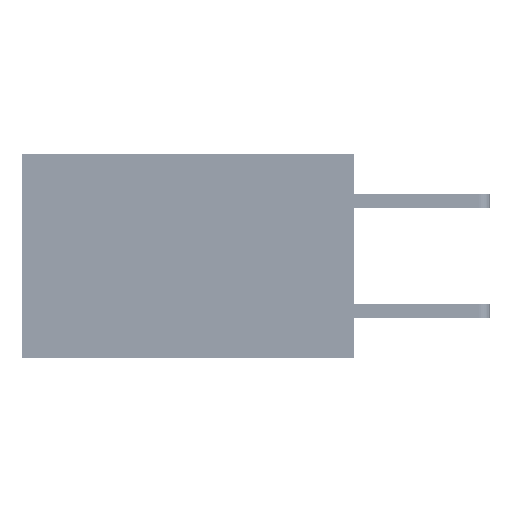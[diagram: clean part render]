
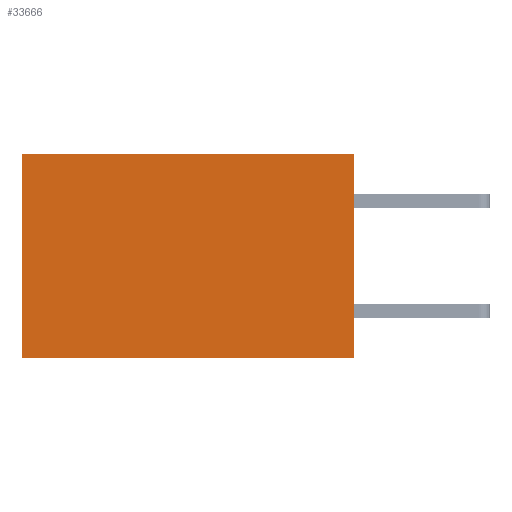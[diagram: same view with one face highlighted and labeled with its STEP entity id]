
A CAD part, left-side view. The second image highlights one B-rep face of the part: STEP entity #33666.
In plain terms, the highlighted planar face has unit normal (-1, 0, 0).
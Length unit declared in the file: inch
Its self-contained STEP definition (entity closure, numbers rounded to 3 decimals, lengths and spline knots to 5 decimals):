
#2239 = EDGE_CURVE ( 'NONE', #25159, #16128, #25951, .T. ) ;
#2943 = AXIS2_PLACEMENT_3D ( 'NONE', #47793, #18213, #14325 ) ;
#3697 = CARTESIAN_POINT ( 'NONE',  ( 0.2875, 0., 0. ) ) ;
#3745 = CARTESIAN_POINT ( 'NONE',  ( 0.2875, 0.6, 0. ) ) ;
#5160 = ORIENTED_EDGE ( 'NONE', *, *, #27192, .T. ) ;
#6220 = VERTEX_POINT ( 'NONE', #3697 ) ;
#8939 = ORIENTED_EDGE ( 'NONE', *, *, #11857, .T. ) ;
#9213 = FACE_OUTER_BOUND ( 'NONE', #27190, .T. ) ;
#11317 = DIRECTION ( 'NONE',  ( 0., 1., 0. ) ) ;
#11857 = EDGE_CURVE ( 'NONE', #6220, #40453, #12612, .T. ) ;
#12612 = LINE ( 'NONE', #37212, #35922 ) ;
#13929 = DIRECTION ( 'NONE',  ( 0., 1., 0. ) ) ;
#14325 = DIRECTION ( 'NONE',  ( 0., 0., -1. ) ) ;
#14468 = VECTOR ( 'NONE', #45276, 39.37008 ) ;
#15050 = CARTESIAN_POINT ( 'NONE',  ( 0.2875, 0., 0. ) ) ;
#16128 = VERTEX_POINT ( 'NONE', #22637 ) ;
#17211 = VECTOR ( 'NONE', #13929, 39.37008 ) ;
#18213 = DIRECTION ( 'NONE',  ( 1., 0., 0. ) ) ;
#21013 = ORIENTED_EDGE ( 'NONE', *, *, #2239, .F. ) ;
#21557 = EDGE_CURVE ( 'NONE', #6220, #25159, #22642, .T. ) ;
#22637 = CARTESIAN_POINT ( 'NONE',  ( 0.2875, 0.6, -0.37 ) ) ;
#22642 = LINE ( 'NONE', #15050, #14468 ) ;
#25159 = VERTEX_POINT ( 'NONE', #44171 ) ;
#25951 = LINE ( 'NONE', #40443, #17211 ) ;
#27190 = EDGE_LOOP ( 'NONE', ( #5160, #21013, #37484, #8939 ) ) ;
#27192 = EDGE_CURVE ( 'NONE', #40453, #16128, #34489, .T. ) ;
#29317 = PLANE ( 'NONE',  #2943 ) ;
#33666 = ADVANCED_FACE ( 'NONE', ( #9213 ), #29317, .F. ) ;
#33918 = VECTOR ( 'NONE', #45382, 39.37008 ) ;
#34489 = LINE ( 'NONE', #42140, #33918 ) ;
#35922 = VECTOR ( 'NONE', #11317, 39.37008 ) ;
#37212 = CARTESIAN_POINT ( 'NONE',  ( 0.2875, 0., 0. ) ) ;
#37484 = ORIENTED_EDGE ( 'NONE', *, *, #21557, .F. ) ;
#40443 = CARTESIAN_POINT ( 'NONE',  ( 0.2875, 0., -0.37 ) ) ;
#40453 = VERTEX_POINT ( 'NONE', #3745 ) ;
#42140 = CARTESIAN_POINT ( 'NONE',  ( 0.2875, 0.6, 0. ) ) ;
#44171 = CARTESIAN_POINT ( 'NONE',  ( 0.2875, 0., -0.37 ) ) ;
#45276 = DIRECTION ( 'NONE',  ( 0., 0., -1. ) ) ;
#45382 = DIRECTION ( 'NONE',  ( 0., 0., -1. ) ) ;
#47793 = CARTESIAN_POINT ( 'NONE',  ( 0.2875, 0., 0. ) ) ;
